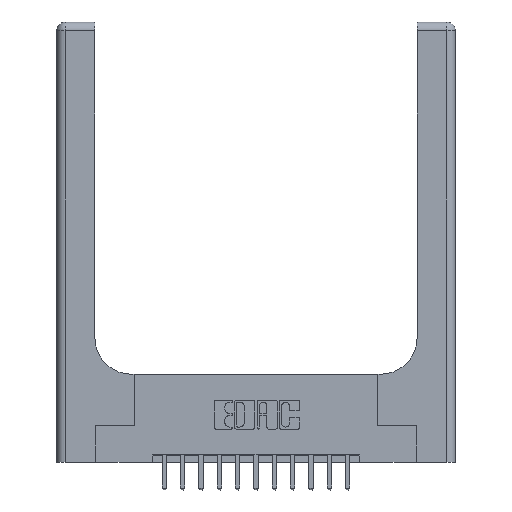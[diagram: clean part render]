
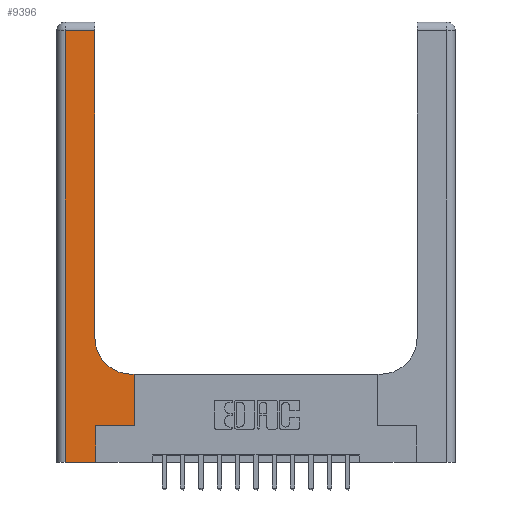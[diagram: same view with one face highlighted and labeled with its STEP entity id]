
A CAD part, top view. The second image highlights one B-rep face of the part: STEP entity #9396.
In plain terms, the highlighted planar face has unit normal (0, 0, 1).
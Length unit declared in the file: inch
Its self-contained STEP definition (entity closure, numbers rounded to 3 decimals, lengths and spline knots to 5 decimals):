
#42 = ORIENTED_EDGE ( 'NONE', *, *, #12981, .T. ) ;
#186 = LINE ( 'NONE', #13182, #942 ) ;
#194 = DIRECTION ( 'NONE',  ( 0., 1., 0. ) ) ;
#409 = AXIS2_PLACEMENT_3D ( 'NONE', #14551, #15669, #2419 ) ;
#695 = EDGE_CURVE ( 'NONE', #1472, #8480, #186, .T. ) ;
#816 = DIRECTION ( 'NONE',  ( 1., 0., 0. ) ) ;
#864 = CARTESIAN_POINT ( 'NONE',  ( 0.265, 0., 0.37 ) ) ;
#942 = VECTOR ( 'NONE', #6573, 39.37008 ) ;
#1005 = CARTESIAN_POINT ( 'NONE',  ( 0.265, 0., 0.37 ) ) ;
#1472 = VERTEX_POINT ( 'NONE', #6686 ) ;
#2121 = ORIENTED_EDGE ( 'NONE', *, *, #4422, .T. ) ;
#2129 = CARTESIAN_POINT ( 'NONE',  ( 0., 0., 0.37 ) ) ;
#2222 = CARTESIAN_POINT ( 'NONE',  ( 0.528, 0.6, 0.37 ) ) ;
#2253 = VERTEX_POINT ( 'NONE', #12823 ) ;
#2419 = DIRECTION ( 'NONE',  ( -1., 0., 0. ) ) ;
#2533 = ORIENTED_EDGE ( 'NONE', *, *, #14089, .T. ) ;
#2681 = ORIENTED_EDGE ( 'NONE', *, *, #3536, .T. ) ;
#2778 = CARTESIAN_POINT ( 'NONE',  ( 0.26, 3., 0.37 ) ) ;
#3134 = CARTESIAN_POINT ( 'NONE',  ( 0.26, 0.6, 0.37 ) ) ;
#3271 = VECTOR ( 'NONE', #14271, 39.37008 ) ;
#3306 = CARTESIAN_POINT ( 'NONE',  ( 0.51, 0.85, 0.37 ) ) ;
#3536 = EDGE_CURVE ( 'NONE', #8480, #13006, #12129, .T. ) ;
#3845 = CIRCLE ( 'NONE', #13539, 0.25 ) ;
#3916 = LINE ( 'NONE', #4010, #8900 ) ;
#4010 = CARTESIAN_POINT ( 'NONE',  ( 0., 2.94, 0.37 ) ) ;
#4142 = FACE_OUTER_BOUND ( 'NONE', #11525, .T. ) ;
#4176 = VECTOR ( 'NONE', #9260, 39.37008 ) ;
#4422 = EDGE_CURVE ( 'NONE', #2253, #4784, #3916, .T. ) ;
#4663 = LINE ( 'NONE', #5980, #11314 ) ;
#4734 = VERTEX_POINT ( 'NONE', #864 ) ;
#4784 = VERTEX_POINT ( 'NONE', #9011 ) ;
#5473 = ORIENTED_EDGE ( 'NONE', *, *, #12406, .T. ) ;
#5980 = CARTESIAN_POINT ( 'NONE',  ( 0.06, 3., 0.37 ) ) ;
#6115 = CARTESIAN_POINT ( 'NONE',  ( 0.265, 0.25, 0.37 ) ) ;
#6298 = VERTEX_POINT ( 'NONE', #7359 ) ;
#6573 = DIRECTION ( 'NONE',  ( 0., 1., 0. ) ) ;
#6686 = CARTESIAN_POINT ( 'NONE',  ( 0.528, 0.25, 0.37 ) ) ;
#7320 = LINE ( 'NONE', #2129, #8271 ) ;
#7359 = CARTESIAN_POINT ( 'NONE',  ( 0.265, 0.25, 0.37 ) ) ;
#8008 = VECTOR ( 'NONE', #15313, 39.37008 ) ;
#8271 = VECTOR ( 'NONE', #816, 39.37008 ) ;
#8480 = VERTEX_POINT ( 'NONE', #2222 ) ;
#8544 = VECTOR ( 'NONE', #194, 39.37008 ) ;
#8900 = VECTOR ( 'NONE', #9300, 39.37008 ) ;
#9011 = CARTESIAN_POINT ( 'NONE',  ( 0.06, 2.94, 0.37 ) ) ;
#9260 = DIRECTION ( 'NONE',  ( -1., 0., 0. ) ) ;
#9300 = DIRECTION ( 'NONE',  ( -1., 0., 0. ) ) ;
#9396 = ADVANCED_FACE ( 'NONE', ( #4142 ), #12999, .F. ) ;
#9753 = CARTESIAN_POINT ( 'NONE',  ( 0.51, 0.6, 0.37 ) ) ;
#9802 = DIRECTION ( 'NONE',  ( 0., -1., 0. ) ) ;
#9902 = DIRECTION ( 'NONE',  ( 1., 0., 0. ) ) ;
#9903 = ORIENTED_EDGE ( 'NONE', *, *, #695, .T. ) ;
#11116 = ORIENTED_EDGE ( 'NONE', *, *, #14001, .T. ) ;
#11284 = DIRECTION ( 'NONE',  ( 0., 0., -1. ) ) ;
#11314 = VECTOR ( 'NONE', #9802, 39.37008 ) ;
#11525 = EDGE_LOOP ( 'NONE', ( #11116, #2121, #2533, #16395, #42, #16968, #9903, #2681, #5473 ) ) ;
#12069 = LINE ( 'NONE', #2778, #8544 ) ;
#12107 = EDGE_CURVE ( 'NONE', #14959, #4734, #7320, .T. ) ;
#12129 = LINE ( 'NONE', #3134, #4176 ) ;
#12406 = EDGE_CURVE ( 'NONE', #13006, #16073, #3845, .T. ) ;
#12823 = CARTESIAN_POINT ( 'NONE',  ( 0.26, 2.94, 0.37 ) ) ;
#12981 = EDGE_CURVE ( 'NONE', #4734, #6298, #13053, .T. ) ;
#12999 = PLANE ( 'NONE',  #409 ) ;
#13006 = VERTEX_POINT ( 'NONE', #9753 ) ;
#13053 = LINE ( 'NONE', #1005, #3271 ) ;
#13182 = CARTESIAN_POINT ( 'NONE',  ( 0.528, 0.25, 0.37 ) ) ;
#13539 = AXIS2_PLACEMENT_3D ( 'NONE', #3306, #11284, #9902 ) ;
#14001 = EDGE_CURVE ( 'NONE', #16073, #2253, #12069, .T. ) ;
#14089 = EDGE_CURVE ( 'NONE', #4784, #14959, #4663, .T. ) ;
#14271 = DIRECTION ( 'NONE',  ( 0., 1., 0. ) ) ;
#14551 = CARTESIAN_POINT ( 'NONE',  ( 0., 3., 0.37 ) ) ;
#14592 = LINE ( 'NONE', #6115, #8008 ) ;
#14736 = EDGE_CURVE ( 'NONE', #6298, #1472, #14592, .T. ) ;
#14959 = VERTEX_POINT ( 'NONE', #16393 ) ;
#15293 = CARTESIAN_POINT ( 'NONE',  ( 0.26, 0.85, 0.37 ) ) ;
#15313 = DIRECTION ( 'NONE',  ( 1., 0., 0. ) ) ;
#15669 = DIRECTION ( 'NONE',  ( 0., 0., -1. ) ) ;
#16073 = VERTEX_POINT ( 'NONE', #15293 ) ;
#16393 = CARTESIAN_POINT ( 'NONE',  ( 0.06, 0., 0.37 ) ) ;
#16395 = ORIENTED_EDGE ( 'NONE', *, *, #12107, .T. ) ;
#16968 = ORIENTED_EDGE ( 'NONE', *, *, #14736, .T. ) ;
